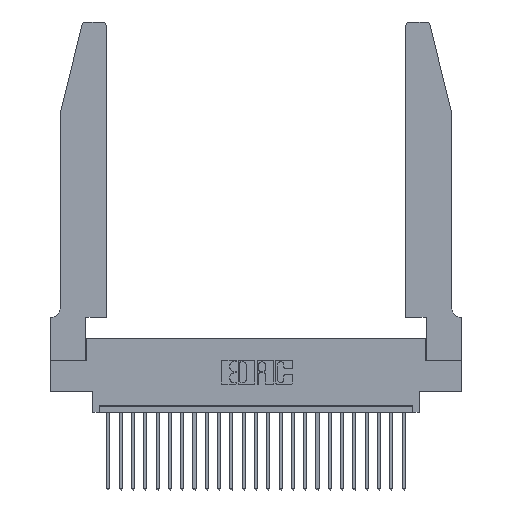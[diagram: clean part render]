
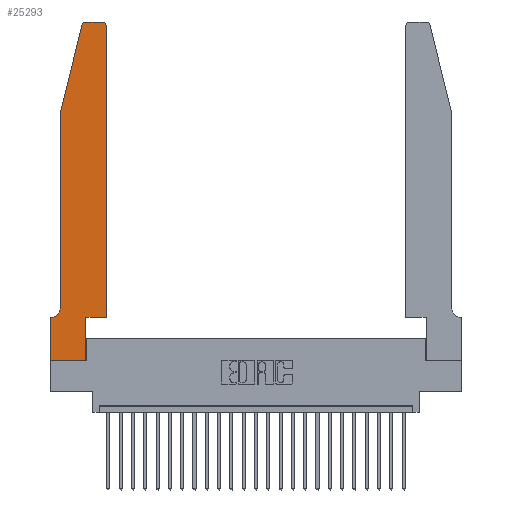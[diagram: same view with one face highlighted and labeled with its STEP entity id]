
A CAD part, top view. The second image highlights one B-rep face of the part: STEP entity #25293.
In plain terms, the highlighted planar face has unit normal (0, 0, 1).
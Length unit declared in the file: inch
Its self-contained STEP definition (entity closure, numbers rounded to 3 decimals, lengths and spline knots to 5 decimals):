
#251 = LINE ( 'NONE', #8716, #24124 ) ;
#702 = PLANE ( 'NONE',  #19238 ) ;
#913 = FACE_OUTER_BOUND ( 'NONE', #5293, .T. ) ;
#966 = ORIENTED_EDGE ( 'NONE', *, *, #7917, .T. ) ;
#1501 = VERTEX_POINT ( 'NONE', #9624 ) ;
#1830 = CARTESIAN_POINT ( 'NONE',  ( 0.0755, 2., 0.37 ) ) ;
#2804 = ORIENTED_EDGE ( 'NONE', *, *, #16025, .T. ) ;
#2896 = CARTESIAN_POINT ( 'NONE',  ( 0.0055, 0.42, 0.37 ) ) ;
#2962 = LINE ( 'NONE', #25673, #4844 ) ;
#3313 = VERTEX_POINT ( 'NONE', #21490 ) ;
#3520 = CARTESIAN_POINT ( 'NONE',  ( 0., 0., 0.37 ) ) ;
#4245 = VERTEX_POINT ( 'NONE', #12486 ) ;
#4423 = CARTESIAN_POINT ( 'NONE',  ( 0.2865, 0., 0.37 ) ) ;
#4436 = DIRECTION ( 'NONE',  ( 1., 0., 0. ) ) ;
#4844 = VECTOR ( 'NONE', #24066, 39.37008 ) ;
#5015 = CARTESIAN_POINT ( 'NONE',  ( 0.4205, 2.72, 0.37 ) ) ;
#5150 = DIRECTION ( 'NONE',  ( -1., 0., 0. ) ) ;
#5293 = EDGE_LOOP ( 'NONE', ( #18268, #966, #24428, #25021, #11897, #5315, #6841, #12760, #19352, #25466, #10614, #2804 ) ) ;
#5315 = ORIENTED_EDGE ( 'NONE', *, *, #9498, .T. ) ;
#5463 = AXIS2_PLACEMENT_3D ( 'NONE', #18348, #20254, #4436 ) ;
#5692 = DIRECTION ( 'NONE',  ( 1., 0., 0. ) ) ;
#5708 = CARTESIAN_POINT ( 'NONE',  ( 0., 0.35, 0.37 ) ) ;
#5773 = LINE ( 'NONE', #8645, #9883 ) ;
#6210 = VERTEX_POINT ( 'NONE', #12286 ) ;
#6308 = EDGE_CURVE ( 'NONE', #16315, #22119, #251, .T. ) ;
#6841 = ORIENTED_EDGE ( 'NONE', *, *, #12289, .T. ) ;
#6905 = LINE ( 'NONE', #8952, #7550 ) ;
#7048 = CARTESIAN_POINT ( 'NONE',  ( 0.4505, 0.35, 0.37 ) ) ;
#7053 = CARTESIAN_POINT ( 'NONE',  ( 0.284, 2.75, 0.37 ) ) ;
#7419 = LINE ( 'NONE', #16649, #16190 ) ;
#7550 = VECTOR ( 'NONE', #9027, 39.37008 ) ;
#7570 = VERTEX_POINT ( 'NONE', #12609 ) ;
#7917 = EDGE_CURVE ( 'NONE', #20102, #16315, #23375, .T. ) ;
#8489 = DIRECTION ( 'NONE',  ( 1., 0., 0. ) ) ;
#8645 = CARTESIAN_POINT ( 'NONE',  ( 0.2865, 0.35, 0.37 ) ) ;
#8716 = CARTESIAN_POINT ( 'NONE',  ( 0.0755, 2., 0.37 ) ) ;
#8788 = VERTEX_POINT ( 'NONE', #22815 ) ;
#8930 = CARTESIAN_POINT ( 'NONE',  ( 0.4505, 0.35, 0.37 ) ) ;
#8952 = CARTESIAN_POINT ( 'NONE',  ( 0.0755, 2., 0.37 ) ) ;
#9027 = DIRECTION ( 'NONE',  ( 0., -1., 0. ) ) ;
#9096 = CARTESIAN_POINT ( 'NONE',  ( 0.0755, 0.42, 0.37 ) ) ;
#9498 = EDGE_CURVE ( 'NONE', #3313, #11394, #2962, .T. ) ;
#9624 = CARTESIAN_POINT ( 'NONE',  ( 0.4505, 0.35, 0.37 ) ) ;
#9883 = VECTOR ( 'NONE', #20643, 39.37008 ) ;
#10394 = CARTESIAN_POINT ( 'NONE',  ( 0., 0.35, 0.37 ) ) ;
#10614 = ORIENTED_EDGE ( 'NONE', *, *, #11828, .T. ) ;
#10828 = VECTOR ( 'NONE', #13340, 39.37008 ) ;
#11394 = VERTEX_POINT ( 'NONE', #5708 ) ;
#11405 = VECTOR ( 'NONE', #8489, 39.37008 ) ;
#11828 = EDGE_CURVE ( 'NONE', #1501, #6210, #16441, .T. ) ;
#11897 = ORIENTED_EDGE ( 'NONE', *, *, #25011, .T. ) ;
#12286 = CARTESIAN_POINT ( 'NONE',  ( 0.4505, 2.72, 0.37 ) ) ;
#12289 = EDGE_CURVE ( 'NONE', #11394, #7570, #23580, .T. ) ;
#12407 = CARTESIAN_POINT ( 'NONE',  ( 0., 0., 0.37 ) ) ;
#12486 = CARTESIAN_POINT ( 'NONE',  ( 0.2865, 0.35, 0.37 ) ) ;
#12609 = CARTESIAN_POINT ( 'NONE',  ( 0., 0., 0.37 ) ) ;
#12739 = VECTOR ( 'NONE', #15614, 39.37008 ) ;
#12747 = EDGE_CURVE ( 'NONE', #4245, #1501, #20086, .T. ) ;
#12760 = ORIENTED_EDGE ( 'NONE', *, *, #22743, .T. ) ;
#13083 = VERTEX_POINT ( 'NONE', #4423 ) ;
#13340 = DIRECTION ( 'NONE',  ( 0., 1., 0. ) ) ;
#13599 = AXIS2_PLACEMENT_3D ( 'NONE', #5015, #23908, #5692 ) ;
#14562 = DIRECTION ( 'NONE',  ( 0., 0., 1. ) ) ;
#14708 = DIRECTION ( 'NONE',  ( -1., 0., 0. ) ) ;
#15614 = DIRECTION ( 'NONE',  ( 1., 0., 0. ) ) ;
#16025 = EDGE_CURVE ( 'NONE', #6210, #8788, #23679, .T. ) ;
#16190 = VECTOR ( 'NONE', #14708, 39.37008 ) ;
#16315 = VERTEX_POINT ( 'NONE', #17209 ) ;
#16438 = DIRECTION ( 'NONE',  ( 0., -1., 0. ) ) ;
#16441 = LINE ( 'NONE', #8930, #10828 ) ;
#16649 = CARTESIAN_POINT ( 'NONE',  ( 0.2605, 2.75, 0.37 ) ) ;
#16742 = VERTEX_POINT ( 'NONE', #9096 ) ;
#17070 = EDGE_CURVE ( 'NONE', #8788, #20102, #7419, .T. ) ;
#17080 = DIRECTION ( 'NONE',  ( 0., 0., -1. ) ) ;
#17090 = AXIS2_PLACEMENT_3D ( 'NONE', #2896, #17080, #5150 ) ;
#17209 = CARTESIAN_POINT ( 'NONE',  ( 0.25487, 2.72718, 0.37 ) ) ;
#17670 = EDGE_CURVE ( 'NONE', #13083, #4245, #5773, .T. ) ;
#18102 = DIRECTION ( 'NONE',  ( -0.239, -0.971, 0. ) ) ;
#18268 = ORIENTED_EDGE ( 'NONE', *, *, #17070, .T. ) ;
#18348 = CARTESIAN_POINT ( 'NONE',  ( 0.284, 2.72, 0.37 ) ) ;
#19238 = AXIS2_PLACEMENT_3D ( 'NONE', #10394, #14562, #22422 ) ;
#19252 = LINE ( 'NONE', #3520, #12739 ) ;
#19352 = ORIENTED_EDGE ( 'NONE', *, *, #17670, .T. ) ;
#20079 = EDGE_CURVE ( 'NONE', #22119, #16742, #6905, .T. ) ;
#20086 = LINE ( 'NONE', #7048, #11405 ) ;
#20102 = VERTEX_POINT ( 'NONE', #7053 ) ;
#20254 = DIRECTION ( 'NONE',  ( 0., 0., 1. ) ) ;
#20643 = DIRECTION ( 'NONE',  ( 0., 1., 0. ) ) ;
#21490 = CARTESIAN_POINT ( 'NONE',  ( 0.0055, 0.35, 0.37 ) ) ;
#22119 = VERTEX_POINT ( 'NONE', #1830 ) ;
#22422 = DIRECTION ( 'NONE',  ( 1., 0., 0. ) ) ;
#22743 = EDGE_CURVE ( 'NONE', #7570, #13083, #19252, .T. ) ;
#22815 = CARTESIAN_POINT ( 'NONE',  ( 0.4205, 2.75, 0.37 ) ) ;
#23375 = CIRCLE ( 'NONE', #5463, 0.03 ) ;
#23580 = LINE ( 'NONE', #12407, #24212 ) ;
#23679 = CIRCLE ( 'NONE', #13599, 0.03 ) ;
#23816 = CIRCLE ( 'NONE', #17090, 0.07 ) ;
#23908 = DIRECTION ( 'NONE',  ( 0., 0., 1. ) ) ;
#24066 = DIRECTION ( 'NONE',  ( -1., 0., 0. ) ) ;
#24124 = VECTOR ( 'NONE', #18102, 39.37008 ) ;
#24212 = VECTOR ( 'NONE', #16438, 39.37008 ) ;
#24428 = ORIENTED_EDGE ( 'NONE', *, *, #6308, .T. ) ;
#25011 = EDGE_CURVE ( 'NONE', #16742, #3313, #23816, .T. ) ;
#25021 = ORIENTED_EDGE ( 'NONE', *, *, #20079, .T. ) ;
#25293 = ADVANCED_FACE ( 'NONE', ( #913 ), #702, .T. ) ;
#25466 = ORIENTED_EDGE ( 'NONE', *, *, #12747, .T. ) ;
#25673 = CARTESIAN_POINT ( 'NONE',  ( 0.0755, 0.35, 0.37 ) ) ;
